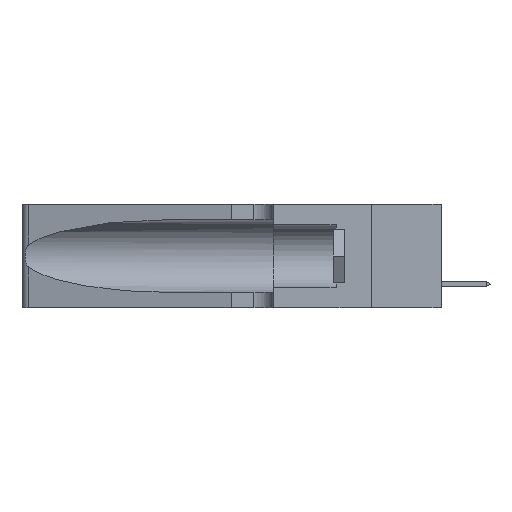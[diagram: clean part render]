
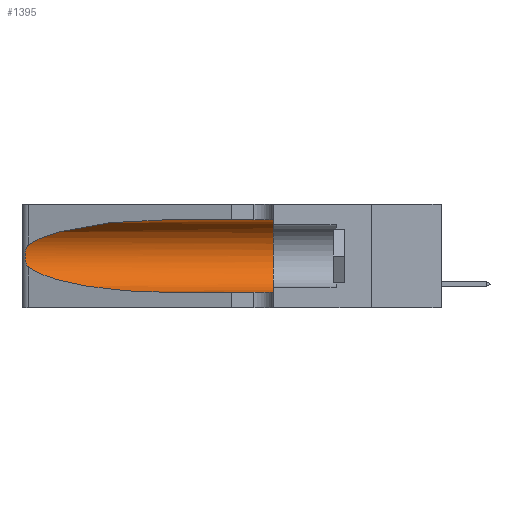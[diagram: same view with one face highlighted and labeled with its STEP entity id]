
A CAD part, left-side view. The second image highlights one B-rep face of the part: STEP entity #1395.
In plain terms, the highlighted cylindrical face has radius 3.308 mm (diameter 6.617 mm), a partial arc.
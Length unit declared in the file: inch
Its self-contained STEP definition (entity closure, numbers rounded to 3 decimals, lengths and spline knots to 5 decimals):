
#147 = CARTESIAN_POINT ( 'NONE',  ( 0.25487, 1.22718, 0.22369 ) ) ;
#201 = ORIENTED_EDGE ( 'NONE', *, *, #17790, .T. ) ;
#502 = VERTEX_POINT ( 'NONE', #21661 ) ;
#1342 = CARTESIAN_POINT ( 'NONE',  ( 0.2373, 1.15595, 0.08982 ) ) ;
#1395 = ADVANCED_FACE ( 'NONE', ( #3918 ), #3625, .F. ) ;
#1745 = CARTESIAN_POINT ( 'NONE',  ( 0.25856, 1.23593, 0.16098 ) ) ;
#1902 = AXIS2_PLACEMENT_3D ( 'NONE', #11198, #14992, #20716 ) ;
#1927 = EDGE_CURVE ( 'NONE', #502, #24061, #2283, .T. ) ;
#1971 = CARTESIAN_POINT ( 'NONE',  ( 0.18966, 0.96281, 0.31525 ) ) ;
#2283 =( BOUNDED_CURVE ( )  B_SPLINE_CURVE ( 3, ( #18458, #1342, #7088, #5231 ),
 .UNSPECIFIED., .F., .T. ) 
 B_SPLINE_CURVE_WITH_KNOTS ( ( 4, 4 ),
 ( 3.44316, 4.71239 ),
 .UNSPECIFIED. ) 
 CURVE ( )  GEOMETRIC_REPRESENTATION_ITEM ( )  RATIONAL_B_SPLINE_CURVE ( ( 1., 0.87, 0.87, 1. ) ) 
 REPRESENTATION_ITEM ( '' )  );
#2930 = CARTESIAN_POINT ( 'NONE',  ( 0.1305, 1.61858, 0.05475 ) ) ;
#3479 = CARTESIAN_POINT ( 'NONE',  ( 0.26018, 1.23835, 0.19895 ) ) ;
#3625 = CYLINDRICAL_SURFACE ( 'NONE', #13119, 0.13025 ) ;
#3743 = CARTESIAN_POINT ( 'NONE',  ( 0.25555, 1.22994, 0.2215 ) ) ;
#3918 = FACE_OUTER_BOUND ( 'NONE', #9007, .T. ) ;
#4995 = ORIENTED_EDGE ( 'NONE', *, *, #6223, .F. ) ;
#5231 = CARTESIAN_POINT ( 'NONE',  ( 0.1305, 0.72297, 0.05475 ) ) ;
#5259 = ORIENTED_EDGE ( 'NONE', *, *, #12932, .T. ) ;
#5865 = CIRCLE ( 'NONE', #1902, 0.13025 ) ;
#6223 = EDGE_CURVE ( 'NONE', #21337, #8401, #18939, .T. ) ;
#6246 =( BOUNDED_CURVE ( )  B_SPLINE_CURVE ( 3, ( #16842, #1971, #13139, #15185 ),
 .UNSPECIFIED., .F., .T. ) 
 B_SPLINE_CURVE_WITH_KNOTS ( ( 4, 4 ),
 ( 1.5708, 2.84003 ),
 .UNSPECIFIED. ) 
 CURVE ( )  GEOMETRIC_REPRESENTATION_ITEM ( )  RATIONAL_B_SPLINE_CURVE ( ( 1., 0.87, 0.87, 1. ) ) 
 REPRESENTATION_ITEM ( '' )  );
#7088 = CARTESIAN_POINT ( 'NONE',  ( 0.18966, 0.96281, 0.05475 ) ) ;
#7564 = LINE ( 'NONE', #2930, #17044 ) ;
#8281 = CARTESIAN_POINT ( 'NONE',  ( 0.1305, 1.61858, 0.185 ) ) ;
#8401 = VERTEX_POINT ( 'NONE', #8914 ) ;
#8914 = CARTESIAN_POINT ( 'NONE',  ( 0.1305, 0.35, 0.31525 ) ) ;
#9007 = EDGE_LOOP ( 'NONE', ( #5259, #11937, #22204, #201, #10385, #4995 ) ) ;
#9183 = CARTESIAN_POINT ( 'NONE',  ( 0.25639, 1.23186, 0.15144 ) ) ;
#9445 = CARTESIAN_POINT ( 'NONE',  ( 0.25487, 1.22718, 0.22369 ) ) ;
#9511 = CARTESIAN_POINT ( 'NONE',  ( 0.1305, 1.61858, 0.31525 ) ) ;
#10385 = ORIENTED_EDGE ( 'NONE', *, *, #15520, .F. ) ;
#10964 = VERTEX_POINT ( 'NONE', #18590 ) ;
#11198 = CARTESIAN_POINT ( 'NONE',  ( 0.1305, 0.35, 0.185 ) ) ;
#11937 = ORIENTED_EDGE ( 'NONE', *, *, #18338, .T. ) ;
#12932 = EDGE_CURVE ( 'NONE', #21337, #20120, #6246, .T. ) ;
#13119 = AXIS2_PLACEMENT_3D ( 'NONE', #8281, #18320, #16310 ) ;
#13139 = CARTESIAN_POINT ( 'NONE',  ( 0.2373, 1.15595, 0.28018 ) ) ;
#13174 = CARTESIAN_POINT ( 'NONE',  ( 0.25639, 1.23184, 0.21858 ) ) ;
#13259 = CARTESIAN_POINT ( 'NONE',  ( 0.26075, 1.23896, 0.178 ) ) ;
#13269 = CARTESIAN_POINT ( 'NONE',  ( 0.1305, 0.72297, 0.31525 ) ) ;
#13336 = CARTESIAN_POINT ( 'NONE',  ( 0.25555, 1.22993, 0.14849 ) ) ;
#13870 = VECTOR ( 'NONE', #18689, 39.37008 ) ;
#13998 = DIRECTION ( 'NONE',  ( 0., -1., 0. ) ) ;
#14888 = CARTESIAN_POINT ( 'NONE',  ( 0.25854, 1.2359, 0.20912 ) ) ;
#14971 = CARTESIAN_POINT ( 'NONE',  ( 0.26017, 1.23833, 0.17102 ) ) ;
#14992 = DIRECTION ( 'NONE',  ( 0., 1., 0. ) ) ;
#15185 = CARTESIAN_POINT ( 'NONE',  ( 0.25487, 1.22718, 0.22369 ) ) ;
#15317 = CARTESIAN_POINT ( 'NONE',  ( 0.1305, 0.72297, 0.05475 ) ) ;
#15520 = EDGE_CURVE ( 'NONE', #8401, #10964, #5865, .T. ) ;
#16310 = DIRECTION ( 'NONE',  ( 0., 0., -1. ) ) ;
#16842 = CARTESIAN_POINT ( 'NONE',  ( 0.1305, 0.72297, 0.31525 ) ) ;
#17044 = VECTOR ( 'NONE', #13998, 39.37008 ) ;
#17499 = B_SPLINE_CURVE_WITH_KNOTS ( 'NONE', 3,
 ( #9445, #3743, #13174, #22606, #14888, #3479, #24419, #13259, #14971, #1745, #22443, #9183, #13336, #24641 ),
 .UNSPECIFIED., .F., .F.,
 ( 4, 2, 2, 2, 2, 2, 4 ),
 ( 0., 0.00027, 0.00053, 0.00107, 0.0016, 0.00187, 0.00214 ),
 .UNSPECIFIED. ) ;
#17790 = EDGE_CURVE ( 'NONE', #24061, #10964, #7564, .T. ) ;
#18320 = DIRECTION ( 'NONE',  ( 0., -1., 0. ) ) ;
#18338 = EDGE_CURVE ( 'NONE', #20120, #502, #17499, .T. ) ;
#18458 = CARTESIAN_POINT ( 'NONE',  ( 0.25487, 1.22718, 0.14631 ) ) ;
#18590 = CARTESIAN_POINT ( 'NONE',  ( 0.1305, 0.35, 0.05475 ) ) ;
#18689 = DIRECTION ( 'NONE',  ( 0., -1., 0. ) ) ;
#18939 = LINE ( 'NONE', #9511, #13870 ) ;
#20120 = VERTEX_POINT ( 'NONE', #147 ) ;
#20716 = DIRECTION ( 'NONE',  ( 0., 0., 1. ) ) ;
#21337 = VERTEX_POINT ( 'NONE', #13269 ) ;
#21661 = CARTESIAN_POINT ( 'NONE',  ( 0.25487, 1.22718, 0.14631 ) ) ;
#22204 = ORIENTED_EDGE ( 'NONE', *, *, #1927, .T. ) ;
#22443 = CARTESIAN_POINT ( 'NONE',  ( 0.25789, 1.23486, 0.15765 ) ) ;
#22606 = CARTESIAN_POINT ( 'NONE',  ( 0.25787, 1.23484, 0.2124 ) ) ;
#24061 = VERTEX_POINT ( 'NONE', #15317 ) ;
#24419 = CARTESIAN_POINT ( 'NONE',  ( 0.26075, 1.23896, 0.19203 ) ) ;
#24641 = CARTESIAN_POINT ( 'NONE',  ( 0.25487, 1.22718, 0.14631 ) ) ;
